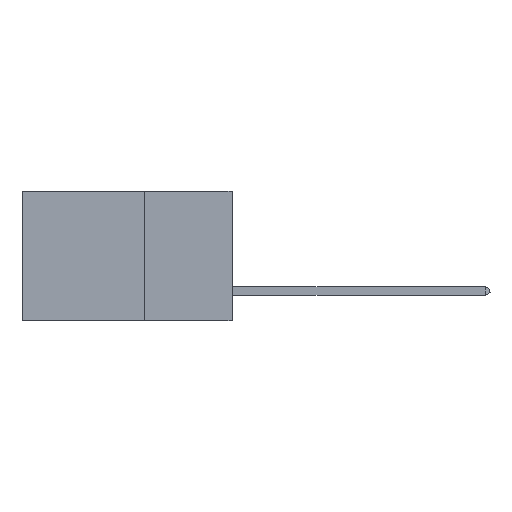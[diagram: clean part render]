
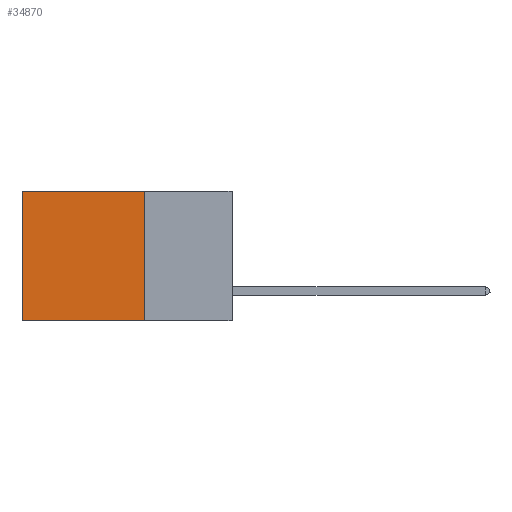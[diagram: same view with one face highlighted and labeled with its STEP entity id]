
A CAD part, left-side view. The second image highlights one B-rep face of the part: STEP entity #34870.
In plain terms, the highlighted planar face has unit normal (-1, 0, 0).
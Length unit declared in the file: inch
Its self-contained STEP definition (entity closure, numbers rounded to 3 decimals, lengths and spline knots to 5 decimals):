
#492 = ORIENTED_EDGE ( 'NONE', *, *, #10914, .T. ) ;
#3318 = FACE_OUTER_BOUND ( 'NONE', #4961, .T. ) ;
#4466 = EDGE_CURVE ( 'NONE', #17836, #39288, #14294, .T. ) ;
#4961 = EDGE_LOOP ( 'NONE', ( #492, #24765, #42384, #31223 ) ) ;
#6091 = DIRECTION ( 'NONE',  ( 0., 1., 0. ) ) ;
#7873 = DIRECTION ( 'NONE',  ( 1., 0., 0. ) ) ;
#8327 = AXIS2_PLACEMENT_3D ( 'NONE', #29734, #7873, #26295 ) ;
#9936 = CARTESIAN_POINT ( 'NONE',  ( 0.2875, 0.25, 0. ) ) ;
#10914 = EDGE_CURVE ( 'NONE', #39288, #36606, #22797, .T. ) ;
#11352 = LINE ( 'NONE', #19376, #24459 ) ;
#13927 = EDGE_CURVE ( 'NONE', #32137, #36606, #11352, .T. ) ;
#14294 = LINE ( 'NONE', #20185, #30606 ) ;
#15439 = DIRECTION ( 'NONE',  ( 0., 1., 0. ) ) ;
#17836 = VERTEX_POINT ( 'NONE', #9936 ) ;
#18418 = PLANE ( 'NONE',  #8327 ) ;
#18949 = CARTESIAN_POINT ( 'NONE',  ( 0.2875, 0.25, 0. ) ) ;
#19376 = CARTESIAN_POINT ( 'NONE',  ( 0.2875, 0.25, -0.37 ) ) ;
#20185 = CARTESIAN_POINT ( 'NONE',  ( 0.2875, 0.25, 0. ) ) ;
#22797 = LINE ( 'NONE', #32787, #42981 ) ;
#24459 = VECTOR ( 'NONE', #15439, 39.37008 ) ;
#24765 = ORIENTED_EDGE ( 'NONE', *, *, #13927, .F. ) ;
#25519 = VECTOR ( 'NONE', #26223, 39.37008 ) ;
#26223 = DIRECTION ( 'NONE',  ( 0., 0., -1. ) ) ;
#26295 = DIRECTION ( 'NONE',  ( 0., 0., -1. ) ) ;
#27805 = LINE ( 'NONE', #18949, #25519 ) ;
#29734 = CARTESIAN_POINT ( 'NONE',  ( 0.2875, 0.25, 0. ) ) ;
#30507 = CARTESIAN_POINT ( 'NONE',  ( 0.2875, 0.6, -0.37 ) ) ;
#30606 = VECTOR ( 'NONE', #6091, 39.37008 ) ;
#31223 = ORIENTED_EDGE ( 'NONE', *, *, #4466, .T. ) ;
#32137 = VERTEX_POINT ( 'NONE', #33006 ) ;
#32787 = CARTESIAN_POINT ( 'NONE',  ( 0.2875, 0.6, 0. ) ) ;
#33006 = CARTESIAN_POINT ( 'NONE',  ( 0.2875, 0.25, -0.37 ) ) ;
#34870 = ADVANCED_FACE ( 'NONE', ( #3318 ), #18418, .F. ) ;
#35925 = DIRECTION ( 'NONE',  ( 0., 0., -1. ) ) ;
#36606 = VERTEX_POINT ( 'NONE', #30507 ) ;
#39288 = VERTEX_POINT ( 'NONE', #43047 ) ;
#42384 = ORIENTED_EDGE ( 'NONE', *, *, #44109, .F. ) ;
#42981 = VECTOR ( 'NONE', #35925, 39.37008 ) ;
#43047 = CARTESIAN_POINT ( 'NONE',  ( 0.2875, 0.6, 0. ) ) ;
#44109 = EDGE_CURVE ( 'NONE', #17836, #32137, #27805, .T. ) ;
